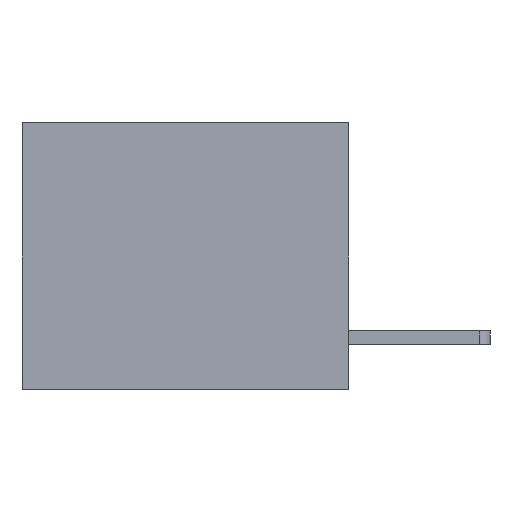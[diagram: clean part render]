
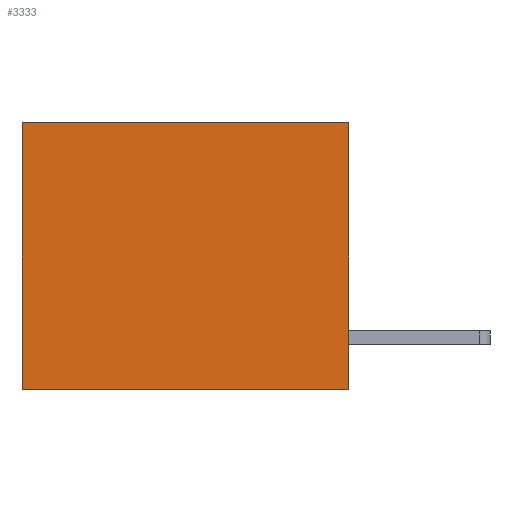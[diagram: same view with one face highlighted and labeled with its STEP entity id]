
A CAD part, left-side view. The second image highlights one B-rep face of the part: STEP entity #3333.
In plain terms, the highlighted planar face has unit normal (-1, 0, 0).
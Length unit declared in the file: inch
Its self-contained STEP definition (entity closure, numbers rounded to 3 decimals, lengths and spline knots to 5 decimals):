
#46 = LINE ( 'NONE', #10505, #7699 ) ;
#339 = ORIENTED_EDGE ( 'NONE', *, *, #4995, .T. ) ;
#353 = EDGE_LOOP ( 'NONE', ( #4350, #7735, #2524, #339 ) ) ;
#883 = VECTOR ( 'NONE', #7455, 39.37008 ) ;
#1329 = CARTESIAN_POINT ( 'NONE',  ( 0.3165, 0., -0.49 ) ) ;
#1673 = CARTESIAN_POINT ( 'NONE',  ( 0.3165, 0., 0. ) ) ;
#1867 = VERTEX_POINT ( 'NONE', #8852 ) ;
#1910 = LINE ( 'NONE', #1673, #6007 ) ;
#2165 = VERTEX_POINT ( 'NONE', #4577 ) ;
#2209 = EDGE_CURVE ( 'NONE', #1867, #6883, #10614, .T. ) ;
#2408 = EDGE_CURVE ( 'NONE', #6883, #2165, #46, .T. ) ;
#2524 = ORIENTED_EDGE ( 'NONE', *, *, #2209, .F. ) ;
#2634 = EDGE_CURVE ( 'NONE', #9413, #2165, #6865, .T. ) ;
#3039 = CARTESIAN_POINT ( 'NONE',  ( 0.3165, 0., -0.49 ) ) ;
#3333 = ADVANCED_FACE ( 'NONE', ( #10741 ), #6559, .F. ) ;
#4350 = ORIENTED_EDGE ( 'NONE', *, *, #2634, .T. ) ;
#4544 = AXIS2_PLACEMENT_3D ( 'NONE', #1329, #9258, #7320 ) ;
#4577 = CARTESIAN_POINT ( 'NONE',  ( 0.3165, 0.6, -0.49 ) ) ;
#4995 = EDGE_CURVE ( 'NONE', #1867, #9413, #1910, .T. ) ;
#6007 = VECTOR ( 'NONE', #7790, 39.37008 ) ;
#6559 = PLANE ( 'NONE',  #4544 ) ;
#6865 = LINE ( 'NONE', #11167, #9510 ) ;
#6883 = VERTEX_POINT ( 'NONE', #7199 ) ;
#6975 = DIRECTION ( 'NONE',  ( 0., 1., 0. ) ) ;
#7199 = CARTESIAN_POINT ( 'NONE',  ( 0.3165, 0., -0.49 ) ) ;
#7320 = DIRECTION ( 'NONE',  ( 0., 0., -1. ) ) ;
#7455 = DIRECTION ( 'NONE',  ( 0., 0., -1. ) ) ;
#7617 = DIRECTION ( 'NONE',  ( 0., 0., -1. ) ) ;
#7699 = VECTOR ( 'NONE', #6975, 39.37008 ) ;
#7735 = ORIENTED_EDGE ( 'NONE', *, *, #2408, .F. ) ;
#7790 = DIRECTION ( 'NONE',  ( 0., 1., 0. ) ) ;
#8852 = CARTESIAN_POINT ( 'NONE',  ( 0.3165, 0., 0. ) ) ;
#9258 = DIRECTION ( 'NONE',  ( 1., 0., 0. ) ) ;
#9413 = VERTEX_POINT ( 'NONE', #10786 ) ;
#9510 = VECTOR ( 'NONE', #7617, 39.37008 ) ;
#10505 = CARTESIAN_POINT ( 'NONE',  ( 0.3165, 0., -0.49 ) ) ;
#10614 = LINE ( 'NONE', #3039, #883 ) ;
#10741 = FACE_OUTER_BOUND ( 'NONE', #353, .T. ) ;
#10786 = CARTESIAN_POINT ( 'NONE',  ( 0.3165, 0.6, 0. ) ) ;
#11167 = CARTESIAN_POINT ( 'NONE',  ( 0.3165, 0.6, -0.49 ) ) ;
